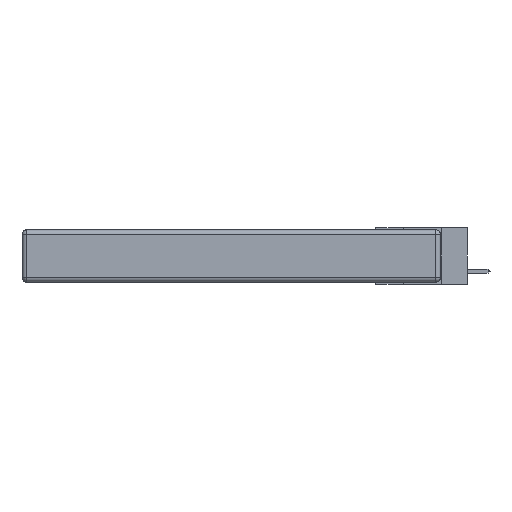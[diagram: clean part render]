
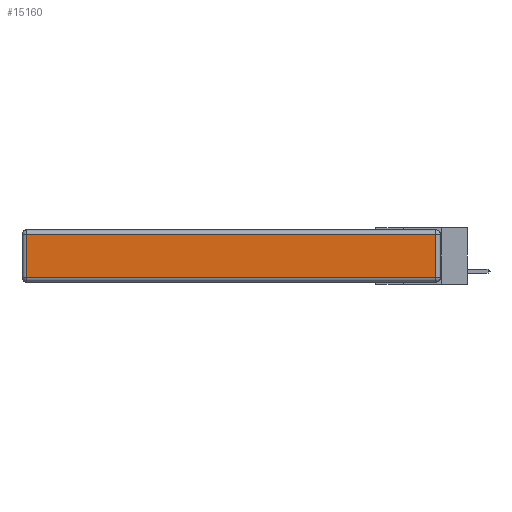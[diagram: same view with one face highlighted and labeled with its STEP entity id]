
A CAD part, left-side view. The second image highlights one B-rep face of the part: STEP entity #15160.
In plain terms, the highlighted planar face has unit normal (-1, 0, 0).
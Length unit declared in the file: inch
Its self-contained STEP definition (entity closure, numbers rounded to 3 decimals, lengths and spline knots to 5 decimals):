
#1073 = EDGE_CURVE ( 'NONE', #7281, #15146, #6406, .T. ) ;
#2198 = DIRECTION ( 'NONE',  ( -1., 0., 0. ) ) ;
#3883 = DIRECTION ( 'NONE',  ( 0., 0., 1. ) ) ;
#4330 = FACE_OUTER_BOUND ( 'NONE', #16398, .T. ) ;
#4905 = ORIENTED_EDGE ( 'NONE', *, *, #16333, .T. ) ;
#6406 = LINE ( 'NONE', #9125, #18812 ) ;
#7269 = VERTEX_POINT ( 'NONE', #11438 ) ;
#7281 = VERTEX_POINT ( 'NONE', #14952 ) ;
#7353 = PLANE ( 'NONE',  #18250 ) ;
#7371 = ORIENTED_EDGE ( 'NONE', *, *, #1073, .T. ) ;
#8887 = ORIENTED_EDGE ( 'NONE', *, *, #14440, .T. ) ;
#9125 = CARTESIAN_POINT ( 'NONE',  ( 0., 0.03, -0.343 ) ) ;
#10417 = LINE ( 'NONE', #13645, #21786 ) ;
#11438 = CARTESIAN_POINT ( 'NONE',  ( 0., 2.72, -0.313 ) ) ;
#12306 = CARTESIAN_POINT ( 'NONE',  ( 0., 0.03, -0.03 ) ) ;
#12813 = VECTOR ( 'NONE', #21749, 39.37008 ) ;
#13064 = LINE ( 'NONE', #14797, #12813 ) ;
#13123 = DIRECTION ( 'NONE',  ( 0., -1., 0. ) ) ;
#13645 = CARTESIAN_POINT ( 'NONE',  ( 0., 2.72, -0.343 ) ) ;
#14440 = EDGE_CURVE ( 'NONE', #15146, #16110, #13064, .T. ) ;
#14471 = ORIENTED_EDGE ( 'NONE', *, *, #14813, .T. ) ;
#14797 = CARTESIAN_POINT ( 'NONE',  ( 0., 2.75, -0.03 ) ) ;
#14813 = EDGE_CURVE ( 'NONE', #16110, #7269, #10417, .T. ) ;
#14952 = CARTESIAN_POINT ( 'NONE',  ( 0., 0.03, -0.313 ) ) ;
#15074 = VECTOR ( 'NONE', #13123, 39.37008 ) ;
#15146 = VERTEX_POINT ( 'NONE', #12306 ) ;
#15160 = ADVANCED_FACE ( 'NONE', ( #4330 ), #7353, .T. ) ;
#15254 = DIRECTION ( 'NONE',  ( 0., 0., -1. ) ) ;
#16110 = VERTEX_POINT ( 'NONE', #19335 ) ;
#16333 = EDGE_CURVE ( 'NONE', #7269, #7281, #19580, .T. ) ;
#16398 = EDGE_LOOP ( 'NONE', ( #4905, #7371, #8887, #14471 ) ) ;
#18250 = AXIS2_PLACEMENT_3D ( 'NONE', #19167, #2198, #3883 ) ;
#18812 = VECTOR ( 'NONE', #20618, 39.37008 ) ;
#19167 = CARTESIAN_POINT ( 'NONE',  ( 0., 0., -0.343 ) ) ;
#19335 = CARTESIAN_POINT ( 'NONE',  ( 0., 2.72, -0.03 ) ) ;
#19580 = LINE ( 'NONE', #21701, #15074 ) ;
#20618 = DIRECTION ( 'NONE',  ( 0., 0., 1. ) ) ;
#21701 = CARTESIAN_POINT ( 'NONE',  ( 0., 0., -0.313 ) ) ;
#21749 = DIRECTION ( 'NONE',  ( 0., 1., 0. ) ) ;
#21786 = VECTOR ( 'NONE', #15254, 39.37008 ) ;
